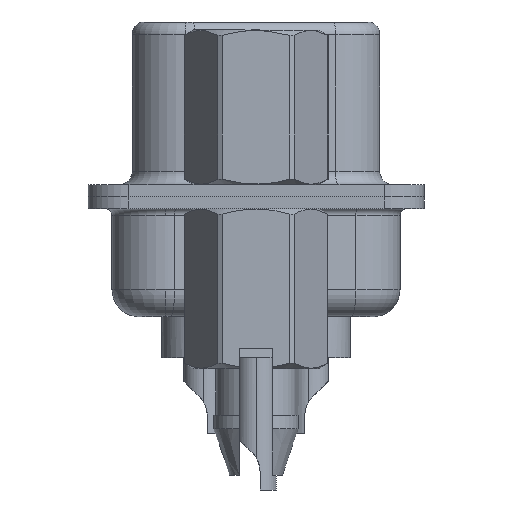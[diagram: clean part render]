
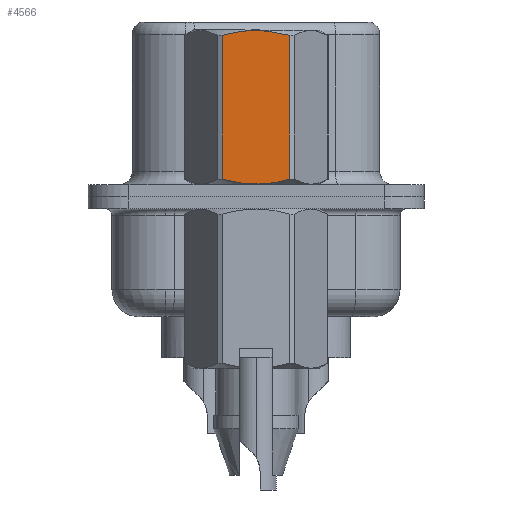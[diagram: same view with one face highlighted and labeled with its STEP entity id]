
A CAD part, left-side view. The second image highlights one B-rep face of the part: STEP entity #4566.
In plain terms, the highlighted planar face has unit normal (-1, 0, 0).
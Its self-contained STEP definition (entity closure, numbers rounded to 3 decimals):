
#33 = CARTESIAN_POINT ( 'NONE',  ( -2.381, -1.273, 3.792 ) ) ;
#634 = VERTEX_POINT ( 'NONE', #23448 ) ;
#1504 = CARTESIAN_POINT ( 'NONE',  ( -2.381, -1.273, 0.652 ) ) ;
#2163 = CARTESIAN_POINT ( 'NONE',  ( -2.381, -0.858, 6.15 ) ) ;
#2309 = CARTESIAN_POINT ( 'NONE',  ( -2.381, 1.273, 6.048 ) ) ;
#3901 = DIRECTION ( 'NONE',  ( 0., 0., -1. ) ) ;
#4566 = ADVANCED_FACE ( 'NONE', ( #28251 ), #7282, .T. ) ;
#5339 = CARTESIAN_POINT ( 'NONE',  ( -2.381, -1.273, 6.048 ) ) ;
#6369 = CARTESIAN_POINT ( 'NONE',  ( -2.381, 0.428, 0.485 ) ) ;
#7282 = PLANE ( 'NONE',  #14917 ) ;
#7287 = ORIENTED_EDGE ( 'NONE', *, *, #23489, .T. ) ;
#7665 = EDGE_CURVE ( 'NONE', #10173, #18975, #26533, .T. ) ;
#7857 = EDGE_LOOP ( 'NONE', ( #7287, #8688, #18257, #18121 ) ) ;
#8290 = EDGE_CURVE ( 'NONE', #25365, #10173, #16508, .T. ) ;
#8598 = CARTESIAN_POINT ( 'NONE',  ( -2.381, 0.215, 6.232 ) ) ;
#8688 = ORIENTED_EDGE ( 'NONE', *, *, #8290, .T. ) ;
#10173 = VERTEX_POINT ( 'NONE', #5339 ) ;
#11015 = CARTESIAN_POINT ( 'NONE',  ( -2.381, 1.065, 0.596 ) ) ;
#11290 = CARTESIAN_POINT ( 'NONE',  ( -2.381, 0.428, 6.215 ) ) ;
#11456 = CARTESIAN_POINT ( 'NONE',  ( -2.381, -0.858, 0.55 ) ) ;
#12643 = VECTOR ( 'NONE', #3901, 1000. ) ;
#13263 = CARTESIAN_POINT ( 'NONE',  ( -2.381, 0.215, 0.468 ) ) ;
#13537 = CARTESIAN_POINT ( 'NONE',  ( -2.381, -1.273, 6.048 ) ) ;
#13685 = CARTESIAN_POINT ( 'NONE',  ( -2.381, -0.432, 6.215 ) ) ;
#13698 = CARTESIAN_POINT ( 'NONE',  ( -2.381, -0.432, 0.485 ) ) ;
#14917 = AXIS2_PLACEMENT_3D ( 'NONE', #27793, #26015, #16438 ) ;
#16102 = CARTESIAN_POINT ( 'NONE',  ( -2.381, -1.273, 0.652 ) ) ;
#16438 = DIRECTION ( 'NONE',  ( 0., -1., 0. ) ) ;
#16508 = LINE ( 'NONE', #33, #16948 ) ;
#16948 = VECTOR ( 'NONE', #25187, 1000. ) ;
#18058 = CARTESIAN_POINT ( 'NONE',  ( -2.381, -0.215, 0.468 ) ) ;
#18121 = ORIENTED_EDGE ( 'NONE', *, *, #20290, .T. ) ;
#18257 = ORIENTED_EDGE ( 'NONE', *, *, #7665, .T. ) ;
#18975 = VERTEX_POINT ( 'NONE', #20062 ) ;
#20004 = CARTESIAN_POINT ( 'NONE',  ( -2.381, 1.065, 6.104 ) ) ;
#20062 = CARTESIAN_POINT ( 'NONE',  ( -2.381, 1.273, 6.048 ) ) ;
#20290 = EDGE_CURVE ( 'NONE', #18975, #634, #29031, .T. ) ;
#20443 = CARTESIAN_POINT ( 'NONE',  ( -2.381, 0.853, 6.151 ) ) ;
#22519 = B_SPLINE_CURVE_WITH_KNOTS ( 'NONE', 3,
 ( #24800, #11015, #29418, #6369, #13263, #18058, #13698, #11456, #25235, #16102 ),
 .UNSPECIFIED., .F., .F.,
 ( 4, 2, 2, 2, 4 ),
 ( 0.003, 0.003, 0.004, 0.004, 0.005 ),
 .UNSPECIFIED. ) ;
#22825 = CARTESIAN_POINT ( 'NONE',  ( -2.381, -1.066, 6.104 ) ) ;
#23448 = CARTESIAN_POINT ( 'NONE',  ( -2.381, 1.273, 0.652 ) ) ;
#23489 = EDGE_CURVE ( 'NONE', #634, #25365, #22519, .T. ) ;
#24419 = CARTESIAN_POINT ( 'NONE',  ( -2.381, 1.273, 3.792 ) ) ;
#24800 = CARTESIAN_POINT ( 'NONE',  ( -2.381, 1.273, 0.652 ) ) ;
#25187 = DIRECTION ( 'NONE',  ( 0., 0., 1. ) ) ;
#25235 = CARTESIAN_POINT ( 'NONE',  ( -2.381, -1.066, 0.596 ) ) ;
#25365 = VERTEX_POINT ( 'NONE', #1504 ) ;
#26015 = DIRECTION ( 'NONE',  ( -1., 0., 0. ) ) ;
#26533 = B_SPLINE_CURVE_WITH_KNOTS ( 'NONE', 3,
 ( #13537, #22825, #2163, #13685, #26882, #8598, #11290, #20443, #20004, #2309 ),
 .UNSPECIFIED., .F., .F.,
 ( 4, 2, 2, 2, 4 ),
 ( 0.001, 0.002, 0.002, 0.003, 0.004 ),
 .UNSPECIFIED. ) ;
#26882 = CARTESIAN_POINT ( 'NONE',  ( -2.381, -0.215, 6.232 ) ) ;
#27793 = CARTESIAN_POINT ( 'NONE',  ( -2.381, 1.375, -3.75 ) ) ;
#28251 = FACE_OUTER_BOUND ( 'NONE', #7857, .T. ) ;
#29031 = LINE ( 'NONE', #24419, #12643 ) ;
#29418 = CARTESIAN_POINT ( 'NONE',  ( -2.381, 0.853, 0.549 ) ) ;
